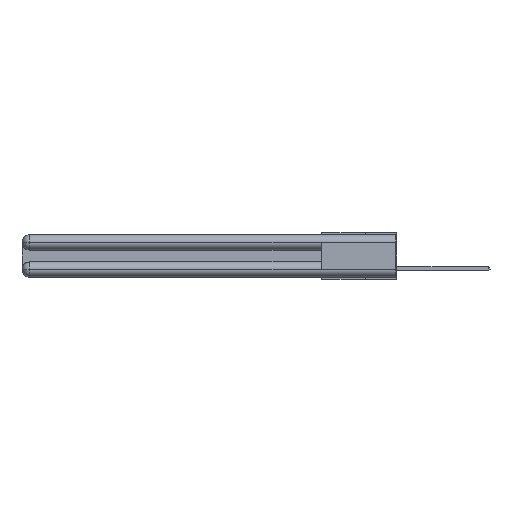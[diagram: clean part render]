
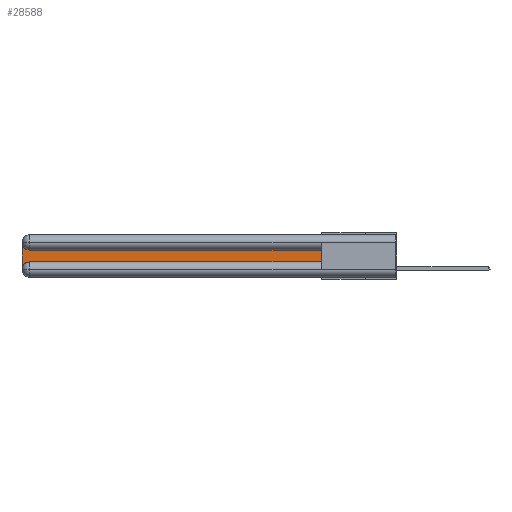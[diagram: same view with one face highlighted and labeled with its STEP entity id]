
A CAD part, left-side view. The second image highlights one B-rep face of the part: STEP entity #28588.
In plain terms, the highlighted planar face has unit normal (-1, 0, 0).
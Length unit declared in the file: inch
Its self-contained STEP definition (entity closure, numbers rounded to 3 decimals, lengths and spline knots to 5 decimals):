
#976 = DIRECTION ( 'NONE',  ( 0., 0., -1. ) ) ;
#1290 = VERTEX_POINT ( 'NONE', #7389 ) ;
#2144 = CARTESIAN_POINT ( 'NONE',  ( 0.075, 0.6, -0.1225 ) ) ;
#2149 = VECTOR ( 'NONE', #11341, 39.37008 ) ;
#2612 = CARTESIAN_POINT ( 'NONE',  ( 0.075, 3., -0.2175 ) ) ;
#3538 = CIRCLE ( 'NONE', #6131, 0.06 ) ;
#4797 = CARTESIAN_POINT ( 'NONE',  ( 0.075, 2.94, -0.2775 ) ) ;
#5423 = LINE ( 'NONE', #2612, #8676 ) ;
#6131 = AXIS2_PLACEMENT_3D ( 'NONE', #25599, #28053, #16505 ) ;
#7108 = DIRECTION ( 'NONE',  ( 0., 0., -1. ) ) ;
#7389 = CARTESIAN_POINT ( 'NONE',  ( 0.075, 3., -0.2775 ) ) ;
#7602 = DIRECTION ( 'NONE',  ( 0., 0., 1. ) ) ;
#7720 = VERTEX_POINT ( 'NONE', #2144 ) ;
#7772 = EDGE_CURVE ( 'NONE', #10899, #7720, #18873, .T. ) ;
#8315 = LINE ( 'NONE', #13470, #2149 ) ;
#8392 = EDGE_CURVE ( 'NONE', #17321, #1290, #5423, .T. ) ;
#8676 = VECTOR ( 'NONE', #13947, 39.37008 ) ;
#8956 = LINE ( 'NONE', #17413, #20547 ) ;
#10127 = DIRECTION ( 'NONE',  ( 0., 1., 0. ) ) ;
#10360 = DIRECTION ( 'NONE',  ( 1., 0., 0. ) ) ;
#10756 = CARTESIAN_POINT ( 'NONE',  ( 0.075, 3., -0.0625 ) ) ;
#10899 = VERTEX_POINT ( 'NONE', #17040 ) ;
#11203 = CARTESIAN_POINT ( 'NONE',  ( 0.075, 2.94, -0.2175 ) ) ;
#11341 = DIRECTION ( 'NONE',  ( 0., -1., 0. ) ) ;
#13470 = CARTESIAN_POINT ( 'NONE',  ( 0.075, 0.6, -0.2175 ) ) ;
#13783 = VECTOR ( 'NONE', #7602, 39.37008 ) ;
#13864 = EDGE_LOOP ( 'NONE', ( #23640, #29601, #20254, #15022, #18332, #26915 ) ) ;
#13947 = DIRECTION ( 'NONE',  ( 0., 0., -1. ) ) ;
#14400 = DIRECTION ( 'NONE',  ( 1., 0., 0. ) ) ;
#14482 = CARTESIAN_POINT ( 'NONE',  ( 0.075, 0.6, -0.2175 ) ) ;
#14827 = CARTESIAN_POINT ( 'NONE',  ( 0.075, 3., -0.1225 ) ) ;
#15022 = ORIENTED_EDGE ( 'NONE', *, *, #29901, .T. ) ;
#16290 = FACE_OUTER_BOUND ( 'NONE', #13864, .T. ) ;
#16294 = VERTEX_POINT ( 'NONE', #23646 ) ;
#16505 = DIRECTION ( 'NONE',  ( 0., 0., -1. ) ) ;
#17040 = CARTESIAN_POINT ( 'NONE',  ( 0.075, 0.6, -0.2175 ) ) ;
#17089 = AXIS2_PLACEMENT_3D ( 'NONE', #14827, #10360, #976 ) ;
#17244 = PLANE ( 'NONE',  #17089 ) ;
#17321 = VERTEX_POINT ( 'NONE', #10756 ) ;
#17413 = CARTESIAN_POINT ( 'NONE',  ( 0.075, 0.6, -0.1225 ) ) ;
#17473 = AXIS2_PLACEMENT_3D ( 'NONE', #4797, #14400, #7108 ) ;
#17760 = VERTEX_POINT ( 'NONE', #11203 ) ;
#18332 = ORIENTED_EDGE ( 'NONE', *, *, #22492, .T. ) ;
#18873 = LINE ( 'NONE', #14482, #13783 ) ;
#20254 = ORIENTED_EDGE ( 'NONE', *, *, #8392, .T. ) ;
#20547 = VECTOR ( 'NONE', #10127, 39.37008 ) ;
#22492 = EDGE_CURVE ( 'NONE', #17760, #10899, #8315, .T. ) ;
#23613 = EDGE_CURVE ( 'NONE', #7720, #16294, #8956, .T. ) ;
#23640 = ORIENTED_EDGE ( 'NONE', *, *, #23613, .T. ) ;
#23646 = CARTESIAN_POINT ( 'NONE',  ( 0.075, 2.94, -0.1225 ) ) ;
#23918 = EDGE_CURVE ( 'NONE', #16294, #17321, #3538, .T. ) ;
#25599 = CARTESIAN_POINT ( 'NONE',  ( 0.075, 2.94, -0.0625 ) ) ;
#26915 = ORIENTED_EDGE ( 'NONE', *, *, #7772, .T. ) ;
#28053 = DIRECTION ( 'NONE',  ( 1., 0., 0. ) ) ;
#28588 = ADVANCED_FACE ( 'NONE', ( #16290 ), #17244, .F. ) ;
#29601 = ORIENTED_EDGE ( 'NONE', *, *, #23918, .T. ) ;
#29901 = EDGE_CURVE ( 'NONE', #1290, #17760, #29952, .T. ) ;
#29952 = CIRCLE ( 'NONE', #17473, 0.06 ) ;
